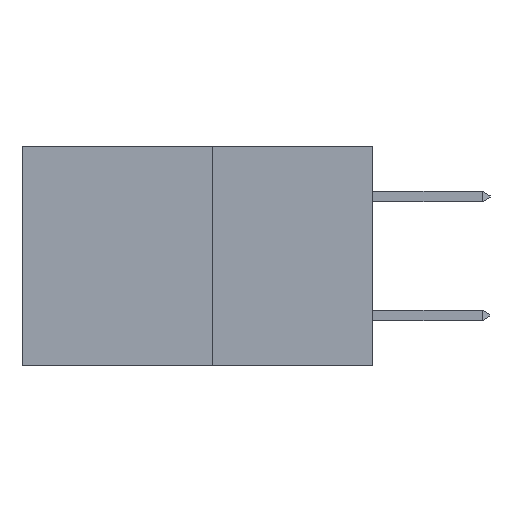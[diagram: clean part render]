
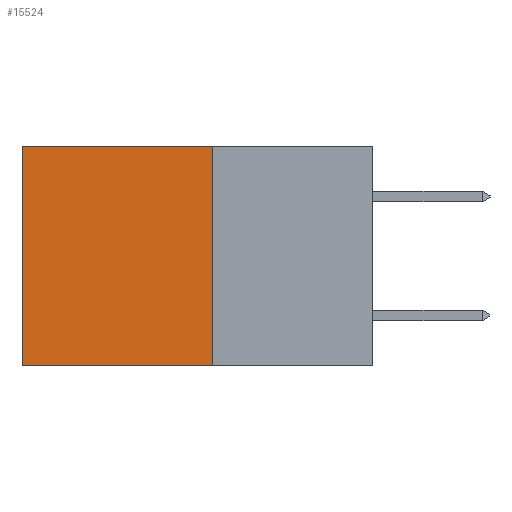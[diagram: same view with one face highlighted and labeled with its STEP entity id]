
A CAD part, left-side view. The second image highlights one B-rep face of the part: STEP entity #15524.
In plain terms, the highlighted planar face has unit normal (-1, 0, 0).
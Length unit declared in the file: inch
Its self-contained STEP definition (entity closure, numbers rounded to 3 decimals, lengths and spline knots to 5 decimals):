
#1575 = VECTOR ( 'NONE', #19068, 39.37008 ) ;
#1738 = CARTESIAN_POINT ( 'NONE',  ( 0.277, 0.27, -0.37 ) ) ;
#4002 = CARTESIAN_POINT ( 'NONE',  ( 0.277, 0.59, -0.37 ) ) ;
#4232 = VERTEX_POINT ( 'NONE', #23030 ) ;
#4350 = CARTESIAN_POINT ( 'NONE',  ( 0.277, 0.59, -0.37 ) ) ;
#4410 = DIRECTION ( 'NONE',  ( 0., 1., 0. ) ) ;
#5190 = PLANE ( 'NONE',  #24583 ) ;
#6750 = ORIENTED_EDGE ( 'NONE', *, *, #14520, .F. ) ;
#7109 = DIRECTION ( 'NONE',  ( 0., 0., -1. ) ) ;
#7171 = FACE_OUTER_BOUND ( 'NONE', #11152, .T. ) ;
#7348 = VERTEX_POINT ( 'NONE', #4350 ) ;
#7657 = LINE ( 'NONE', #21053, #12078 ) ;
#8511 = CARTESIAN_POINT ( 'NONE',  ( 0.277, 0.59, 0. ) ) ;
#10034 = EDGE_CURVE ( 'NONE', #24278, #7348, #11113, .T. ) ;
#10071 = EDGE_CURVE ( 'NONE', #4232, #18807, #15570, .T. ) ;
#11113 = LINE ( 'NONE', #4002, #1575 ) ;
#11152 = EDGE_LOOP ( 'NONE', ( #15606, #6750, #21741, #22328 ) ) ;
#12078 = VECTOR ( 'NONE', #22910, 39.37008 ) ;
#13569 = CARTESIAN_POINT ( 'NONE',  ( 0.277, 0.27, -0.37 ) ) ;
#14520 = EDGE_CURVE ( 'NONE', #18807, #7348, #7657, .T. ) ;
#14611 = EDGE_CURVE ( 'NONE', #4232, #24278, #19733, .T. ) ;
#14745 = VECTOR ( 'NONE', #4410, 39.37008 ) ;
#15524 = ADVANCED_FACE ( 'NONE', ( #7171 ), #5190, .F. ) ;
#15570 = LINE ( 'NONE', #13569, #19974 ) ;
#15606 = ORIENTED_EDGE ( 'NONE', *, *, #10034, .T. ) ;
#18396 = DIRECTION ( 'NONE',  ( 1., 0., 0. ) ) ;
#18807 = VERTEX_POINT ( 'NONE', #1738 ) ;
#19068 = DIRECTION ( 'NONE',  ( 0., 0., -1. ) ) ;
#19733 = LINE ( 'NONE', #21285, #14745 ) ;
#19974 = VECTOR ( 'NONE', #22894, 39.37008 ) ;
#21053 = CARTESIAN_POINT ( 'NONE',  ( 0.277, 0.27, -0.37 ) ) ;
#21285 = CARTESIAN_POINT ( 'NONE',  ( 0.277, 0.27, 0. ) ) ;
#21741 = ORIENTED_EDGE ( 'NONE', *, *, #10071, .F. ) ;
#22328 = ORIENTED_EDGE ( 'NONE', *, *, #14611, .T. ) ;
#22894 = DIRECTION ( 'NONE',  ( 0., 0., -1. ) ) ;
#22910 = DIRECTION ( 'NONE',  ( 0., 1., 0. ) ) ;
#23030 = CARTESIAN_POINT ( 'NONE',  ( 0.277, 0.27, 0. ) ) ;
#23968 = CARTESIAN_POINT ( 'NONE',  ( 0.277, 0.27, -0.37 ) ) ;
#24278 = VERTEX_POINT ( 'NONE', #8511 ) ;
#24583 = AXIS2_PLACEMENT_3D ( 'NONE', #23968, #18396, #7109 ) ;
